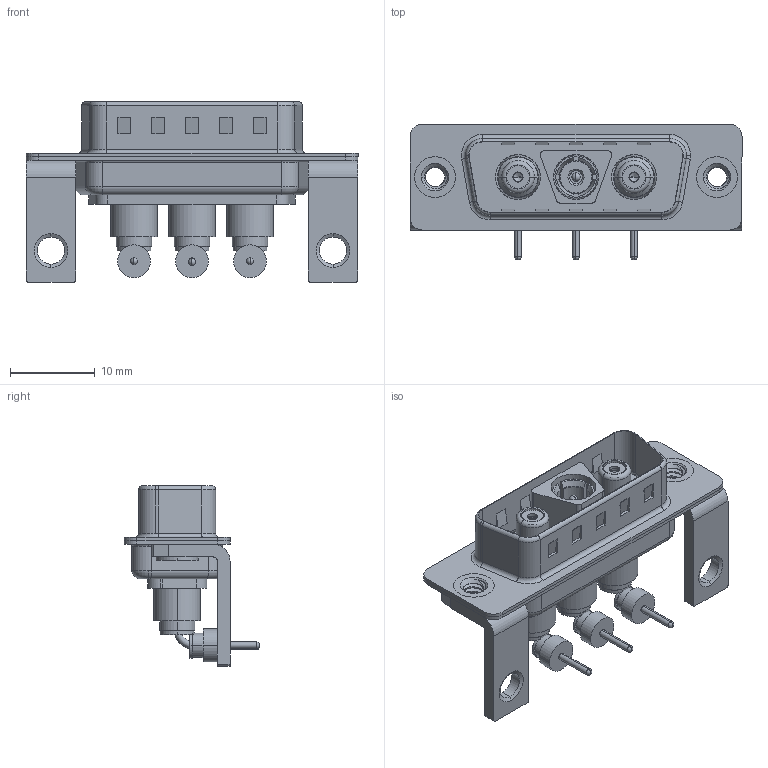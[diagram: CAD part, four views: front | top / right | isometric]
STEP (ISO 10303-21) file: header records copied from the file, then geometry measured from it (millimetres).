
FILE_DESCRIPTION (( 'STEP AP203' ), '1' );
FILE_NAME ('629-3WK3640-5T4.STEP', '2022-05-05T13:56:43', ( '' ), ( '' ), 'SwSTEP 2.0', 'SolidWorks 2020', '' );
FILE_SCHEMA (( 'CONFIG_CONTROL_DESIGN' ));
Length unit declared in the file: millimetre
Products named in the file (18): 629Combo Stabilizer Bracket; Locking Collar; 629Combo Housing_3WK3; Insulator Socket; Socket_RA; Insulator Socket 2; Co-Ax Plug Assy_RA; 629Combo Shell Rear_15 Contacts; 629Combo Threaded Rivet_3; 629-3WK3640-5T4; Co-Ax Jack Assy_RA; Insulator RA Pin; 629Combo Shell Front_15 Contacts; Pin_RA; Co-Ax Plug_RA PC Tail; Co-Ax Jack_RA PC Tail; Insulator Pin_Straight PC Tail
Assembly tree (27 placements, depth 3):
  629-3WK3640-5T4
    629Combo Housing_3WK3
    629Combo Shell Rear_15 Contacts
    629Combo Shell Front_15 Contacts
    629Combo Threaded Rivet_3  x2
    629Combo Stabilizer Bracket  x2
    Co-Ax Plug Assy_RA
      Co-Ax Plug_RA PC Tail
      Insulator Pin_Straight PC Tail
      Pin_RA
      Locking Collar
      Insulator RA Pin
    Co-Ax Jack Assy_RA
      Co-Ax Jack_RA PC Tail
      Insulator Socket
      Insulator Socket 2
      Locking Collar
      Socket_RA
      Insulator RA Pin
    Co-Ax Jack Assy_RA
      Co-Ax Jack_RA PC Tail
      Insulator Socket
      Insulator Socket 2
      Locking Collar
      Socket_RA
      Insulator RA Pin
Bounding box: 39.2 x 16 x 21.3 mm (x, y, z)
Volume: 2542.3 mm3; surface area: 7212.2 mm2
Topology: 24 solids, 24 shells, 757 faces, 1820 edges, 1150 vertices
Faces by surface type: cylinder 337, plane 276, torus 68, cone 59, bspline 9, sphere 8
Entity records: 20557 total; most frequent: CARTESIAN_POINT 4491, DIRECTION 3120, ORIENTED_EDGE 2756, EDGE_CURVE 1378, AXIS2_PLACEMENT_3D 1212, VERTEX_POINT 875, VECTOR 696, LINE 696
